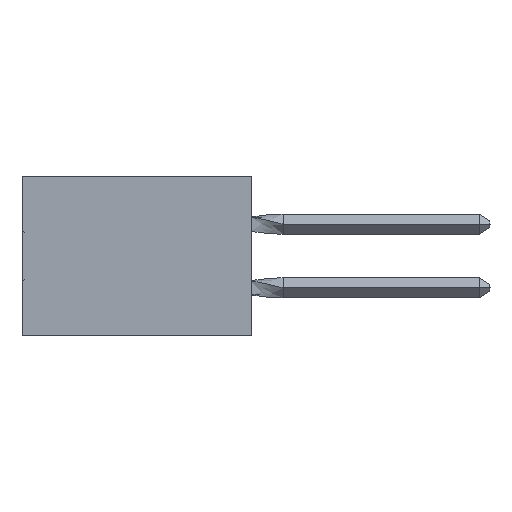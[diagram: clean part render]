
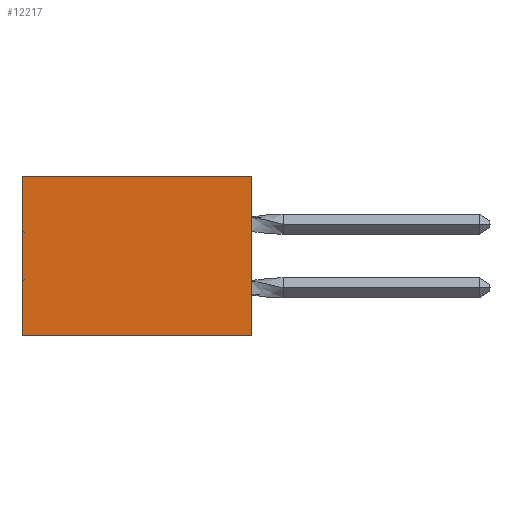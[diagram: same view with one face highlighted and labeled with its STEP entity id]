
A CAD part, left-side view. The second image highlights one B-rep face of the part: STEP entity #12217.
In plain terms, the highlighted planar face has unit normal (-1, 0, 0).
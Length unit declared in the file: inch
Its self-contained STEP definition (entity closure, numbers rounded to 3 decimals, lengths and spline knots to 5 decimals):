
#694 = ORIENTED_EDGE ( 'NONE', *, *, #50197, .T. ) ;
#1492 = FACE_OUTER_BOUND ( 'NONE', #7875, .T. ) ;
#2787 = CARTESIAN_POINT ( 'NONE',  ( 0.305, 0., -0.5 ) ) ;
#2907 = DIRECTION ( 'NONE',  ( 0., 1., 0. ) ) ;
#3105 = VERTEX_POINT ( 'NONE', #9222 ) ;
#4487 = EDGE_CURVE ( 'NONE', #3105, #55239, #49043, .T. ) ;
#7875 = EDGE_LOOP ( 'NONE', ( #694, #26572, #32480, #26475 ) ) ;
#8384 = AXIS2_PLACEMENT_3D ( 'NONE', #12987, #47606, #25803 ) ;
#8672 = VERTEX_POINT ( 'NONE', #47604 ) ;
#9222 = CARTESIAN_POINT ( 'NONE',  ( 0.305, 0., 0. ) ) ;
#9433 = VECTOR ( 'NONE', #43805, 39.37008 ) ;
#10157 = CARTESIAN_POINT ( 'NONE',  ( 0.305, 0.72, -0.5 ) ) ;
#12217 = ADVANCED_FACE ( 'NONE', ( #1492 ), #43272, .F. ) ;
#12841 = DIRECTION ( 'NONE',  ( 0., 0., -1. ) ) ;
#12987 = CARTESIAN_POINT ( 'NONE',  ( 0.305, 0., -0.5 ) ) ;
#13147 = CARTESIAN_POINT ( 'NONE',  ( 0.305, 0., -0.5 ) ) ;
#14282 = VECTOR ( 'NONE', #38498, 39.37008 ) ;
#14981 = EDGE_CURVE ( 'NONE', #3105, #20659, #31894, .T. ) ;
#20659 = VERTEX_POINT ( 'NONE', #2787 ) ;
#21688 = LINE ( 'NONE', #13147, #9433 ) ;
#23835 = LINE ( 'NONE', #10157, #14282 ) ;
#25803 = DIRECTION ( 'NONE',  ( 0., 0., -1. ) ) ;
#26475 = ORIENTED_EDGE ( 'NONE', *, *, #4487, .T. ) ;
#26508 = VECTOR ( 'NONE', #2907, 39.37008 ) ;
#26572 = ORIENTED_EDGE ( 'NONE', *, *, #53831, .F. ) ;
#29118 = CARTESIAN_POINT ( 'NONE',  ( 0.305, 0., 0. ) ) ;
#30911 = CARTESIAN_POINT ( 'NONE',  ( 0.305, 0.72, 0. ) ) ;
#31894 = LINE ( 'NONE', #34825, #55204 ) ;
#32480 = ORIENTED_EDGE ( 'NONE', *, *, #14981, .F. ) ;
#34825 = CARTESIAN_POINT ( 'NONE',  ( 0.305, 0., -0.5 ) ) ;
#38498 = DIRECTION ( 'NONE',  ( 0., 0., -1. ) ) ;
#43272 = PLANE ( 'NONE',  #8384 ) ;
#43805 = DIRECTION ( 'NONE',  ( 0., 1., 0. ) ) ;
#47604 = CARTESIAN_POINT ( 'NONE',  ( 0.305, 0.72, -0.5 ) ) ;
#47606 = DIRECTION ( 'NONE',  ( 1., 0., 0. ) ) ;
#49043 = LINE ( 'NONE', #29118, #26508 ) ;
#50197 = EDGE_CURVE ( 'NONE', #55239, #8672, #23835, .T. ) ;
#53831 = EDGE_CURVE ( 'NONE', #20659, #8672, #21688, .T. ) ;
#55204 = VECTOR ( 'NONE', #12841, 39.37008 ) ;
#55239 = VERTEX_POINT ( 'NONE', #30911 ) ;
